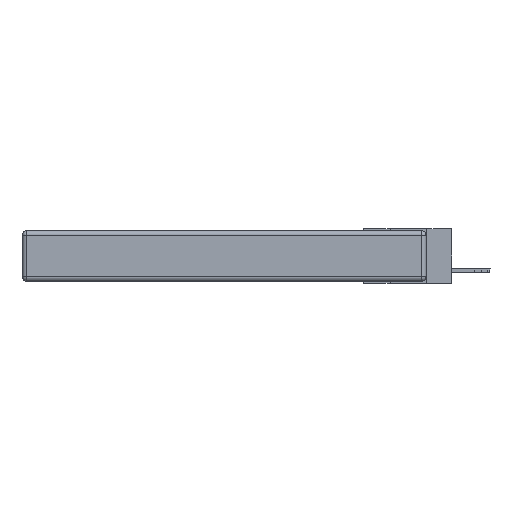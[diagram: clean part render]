
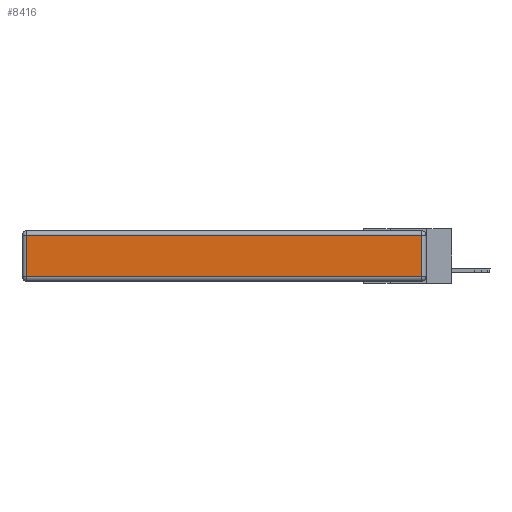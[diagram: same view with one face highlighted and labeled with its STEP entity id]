
A CAD part, left-side view. The second image highlights one B-rep face of the part: STEP entity #8416.
In plain terms, the highlighted planar face has unit normal (-1, 0, 0).
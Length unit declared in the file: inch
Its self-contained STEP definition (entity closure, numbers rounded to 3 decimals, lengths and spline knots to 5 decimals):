
#966 = CARTESIAN_POINT ( 'NONE',  ( 0., 2.72, -0.313 ) ) ;
#1028 = CARTESIAN_POINT ( 'NONE',  ( 0., 0., -0.313 ) ) ;
#1485 = VERTEX_POINT ( 'NONE', #1551 ) ;
#1551 = CARTESIAN_POINT ( 'NONE',  ( 0., 0.03, -0.03 ) ) ;
#1654 = VERTEX_POINT ( 'NONE', #17710 ) ;
#2013 = AXIS2_PLACEMENT_3D ( 'NONE', #19187, #17726, #11473 ) ;
#2709 = DIRECTION ( 'NONE',  ( 0., 0., 1. ) ) ;
#3211 = CARTESIAN_POINT ( 'NONE',  ( 0., 2.72, -0.343 ) ) ;
#3553 = ORIENTED_EDGE ( 'NONE', *, *, #9867, .T. ) ;
#3881 = EDGE_CURVE ( 'NONE', #4722, #12784, #19772, .T. ) ;
#4650 = ORIENTED_EDGE ( 'NONE', *, *, #14924, .T. ) ;
#4722 = VERTEX_POINT ( 'NONE', #966 ) ;
#5141 = CARTESIAN_POINT ( 'NONE',  ( 0., 0.03, -0.313 ) ) ;
#5434 = PLANE ( 'NONE',  #2013 ) ;
#7121 = EDGE_CURVE ( 'NONE', #12784, #1485, #15091, .T. ) ;
#7183 = CARTESIAN_POINT ( 'NONE',  ( 0., 2.75, -0.03 ) ) ;
#7536 = DIRECTION ( 'NONE',  ( 0., -1., 0. ) ) ;
#8416 = ADVANCED_FACE ( 'NONE', ( #18593 ), #5434, .T. ) ;
#8965 = ORIENTED_EDGE ( 'NONE', *, *, #7121, .T. ) ;
#9867 = EDGE_CURVE ( 'NONE', #1485, #1654, #11835, .T. ) ;
#9942 = EDGE_LOOP ( 'NONE', ( #11975, #8965, #3553, #4650 ) ) ;
#10985 = DIRECTION ( 'NONE',  ( 0., 0., -1. ) ) ;
#11016 = VECTOR ( 'NONE', #2709, 39.37008 ) ;
#11473 = DIRECTION ( 'NONE',  ( 0., 0., 1. ) ) ;
#11835 = LINE ( 'NONE', #7183, #17370 ) ;
#11975 = ORIENTED_EDGE ( 'NONE', *, *, #3881, .T. ) ;
#12129 = LINE ( 'NONE', #3211, #18863 ) ;
#12784 = VERTEX_POINT ( 'NONE', #5141 ) ;
#13486 = CARTESIAN_POINT ( 'NONE',  ( 0., 0.03, -0.343 ) ) ;
#14695 = VECTOR ( 'NONE', #7536, 39.37008 ) ;
#14808 = DIRECTION ( 'NONE',  ( 0., 1., 0. ) ) ;
#14924 = EDGE_CURVE ( 'NONE', #1654, #4722, #12129, .T. ) ;
#15091 = LINE ( 'NONE', #13486, #11016 ) ;
#17370 = VECTOR ( 'NONE', #14808, 39.37008 ) ;
#17710 = CARTESIAN_POINT ( 'NONE',  ( 0., 2.72, -0.03 ) ) ;
#17726 = DIRECTION ( 'NONE',  ( -1., 0., 0. ) ) ;
#18593 = FACE_OUTER_BOUND ( 'NONE', #9942, .T. ) ;
#18863 = VECTOR ( 'NONE', #10985, 39.37008 ) ;
#19187 = CARTESIAN_POINT ( 'NONE',  ( 0., 0., -0.343 ) ) ;
#19772 = LINE ( 'NONE', #1028, #14695 ) ;
